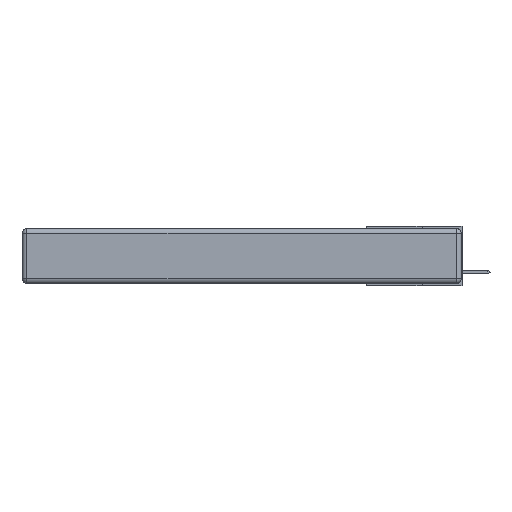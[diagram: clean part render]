
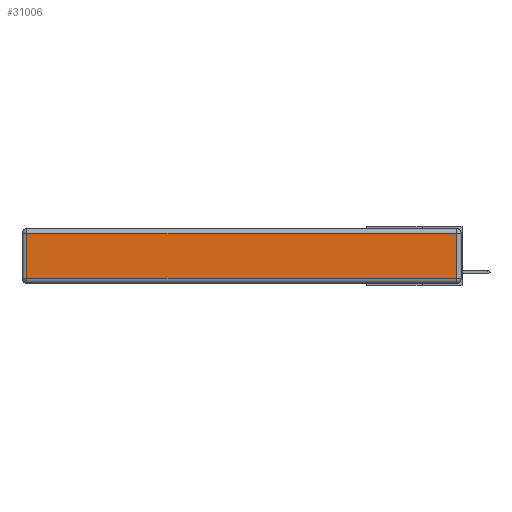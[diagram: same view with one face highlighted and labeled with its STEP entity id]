
A CAD part, left-side view. The second image highlights one B-rep face of the part: STEP entity #31006.
In plain terms, the highlighted planar face has unit normal (-1, 0, 0).
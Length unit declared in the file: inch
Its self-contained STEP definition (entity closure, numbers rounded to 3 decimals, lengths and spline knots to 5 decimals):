
#317 = LINE ( 'NONE', #6595, #17760 ) ;
#395 = ORIENTED_EDGE ( 'NONE', *, *, #8716, .T. ) ;
#857 = ORIENTED_EDGE ( 'NONE', *, *, #6602, .T. ) ;
#1687 = DIRECTION ( 'NONE',  ( 0., 1., 0. ) ) ;
#3994 = CARTESIAN_POINT ( 'NONE',  ( 0., 0., -0.313 ) ) ;
#5007 = CARTESIAN_POINT ( 'NONE',  ( 0., 0.03, -0.313 ) ) ;
#6229 = DIRECTION ( 'NONE',  ( 0., 0., 1. ) ) ;
#6595 = CARTESIAN_POINT ( 'NONE',  ( 0., 2.72, -0.343 ) ) ;
#6602 = EDGE_CURVE ( 'NONE', #12729, #31045, #317, .T. ) ;
#6884 = ORIENTED_EDGE ( 'NONE', *, *, #31800, .T. ) ;
#7935 = CARTESIAN_POINT ( 'NONE',  ( 0., 2.72, -0.313 ) ) ;
#8153 = CARTESIAN_POINT ( 'NONE',  ( 0., 0., -0.343 ) ) ;
#8716 = EDGE_CURVE ( 'NONE', #29489, #12729, #16095, .T. ) ;
#10152 = DIRECTION ( 'NONE',  ( 0., 0., 1. ) ) ;
#11030 = DIRECTION ( 'NONE',  ( 0., 0., -1. ) ) ;
#12515 = ORIENTED_EDGE ( 'NONE', *, *, #21147, .T. ) ;
#12556 = VECTOR ( 'NONE', #13871, 39.37008 ) ;
#12729 = VERTEX_POINT ( 'NONE', #17566 ) ;
#13340 = EDGE_LOOP ( 'NONE', ( #12515, #6884, #395, #857 ) ) ;
#13379 = VECTOR ( 'NONE', #6229, 39.37008 ) ;
#13547 = CARTESIAN_POINT ( 'NONE',  ( 0., 0.03, -0.343 ) ) ;
#13871 = DIRECTION ( 'NONE',  ( 0., -1., 0. ) ) ;
#14524 = LINE ( 'NONE', #3994, #12556 ) ;
#15265 = CARTESIAN_POINT ( 'NONE',  ( 0., 0.03, -0.03 ) ) ;
#16095 = LINE ( 'NONE', #32145, #22054 ) ;
#17566 = CARTESIAN_POINT ( 'NONE',  ( 0., 2.72, -0.03 ) ) ;
#17760 = VECTOR ( 'NONE', #11030, 39.37008 ) ;
#20319 = AXIS2_PLACEMENT_3D ( 'NONE', #8153, #25567, #10152 ) ;
#21147 = EDGE_CURVE ( 'NONE', #31045, #23176, #14524, .T. ) ;
#22054 = VECTOR ( 'NONE', #1687, 39.37008 ) ;
#23176 = VERTEX_POINT ( 'NONE', #5007 ) ;
#23344 = PLANE ( 'NONE',  #20319 ) ;
#25567 = DIRECTION ( 'NONE',  ( -1., 0., 0. ) ) ;
#29489 = VERTEX_POINT ( 'NONE', #15265 ) ;
#29708 = FACE_OUTER_BOUND ( 'NONE', #13340, .T. ) ;
#30014 = LINE ( 'NONE', #13547, #13379 ) ;
#31006 = ADVANCED_FACE ( 'NONE', ( #29708 ), #23344, .T. ) ;
#31045 = VERTEX_POINT ( 'NONE', #7935 ) ;
#31800 = EDGE_CURVE ( 'NONE', #23176, #29489, #30014, .T. ) ;
#32145 = CARTESIAN_POINT ( 'NONE',  ( 0., 2.75, -0.03 ) ) ;
